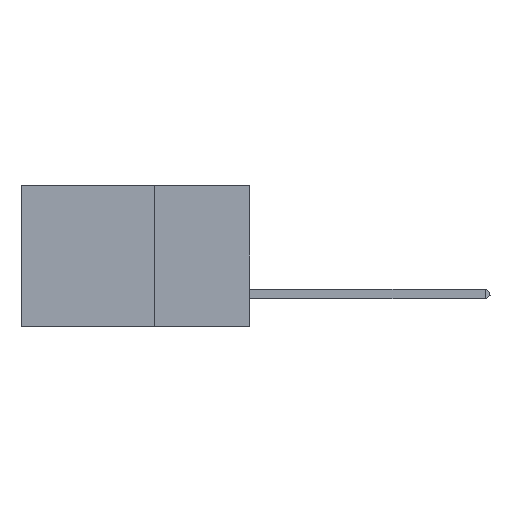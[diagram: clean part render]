
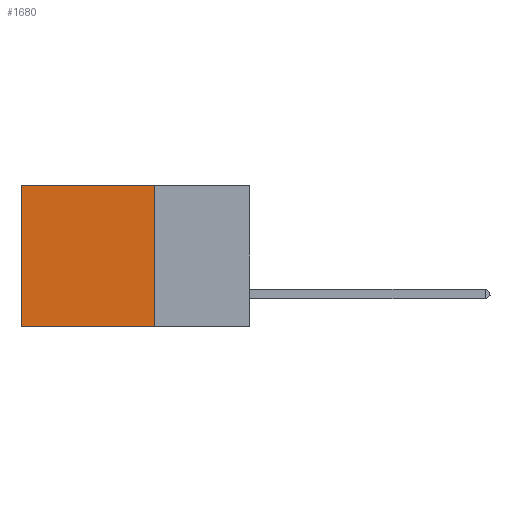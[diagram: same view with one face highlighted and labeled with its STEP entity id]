
A CAD part, left-side view. The second image highlights one B-rep face of the part: STEP entity #1680.
In plain terms, the highlighted planar face has unit normal (-1, 0, 0).
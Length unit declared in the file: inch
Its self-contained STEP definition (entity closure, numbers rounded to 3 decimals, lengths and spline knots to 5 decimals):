
#874 = ORIENTED_EDGE ( 'NONE', *, *, #21182, .F. ) ;
#1271 = CARTESIAN_POINT ( 'NONE',  ( 0.2875, 0.25, 0. ) ) ;
#1680 = ADVANCED_FACE ( 'NONE', ( #31434 ), #6539, .F. ) ;
#3953 = CARTESIAN_POINT ( 'NONE',  ( 0.2875, 0.25, 0. ) ) ;
#4051 = VERTEX_POINT ( 'NONE', #11781 ) ;
#4622 = EDGE_CURVE ( 'NONE', #23610, #4051, #10595, .T. ) ;
#5196 = CARTESIAN_POINT ( 'NONE',  ( 0.2875, 0.25, -0.37 ) ) ;
#5787 = VERTEX_POINT ( 'NONE', #28684 ) ;
#5851 = EDGE_CURVE ( 'NONE', #18109, #5787, #27146, .T. ) ;
#6539 = PLANE ( 'NONE',  #11853 ) ;
#6993 = LINE ( 'NONE', #5196, #16858 ) ;
#8782 = DIRECTION ( 'NONE',  ( 0., 0., -1. ) ) ;
#9508 = DIRECTION ( 'NONE',  ( 1., 0., 0. ) ) ;
#9754 = DIRECTION ( 'NONE',  ( 0., 0., -1. ) ) ;
#10595 = LINE ( 'NONE', #11895, #27715 ) ;
#11781 = CARTESIAN_POINT ( 'NONE',  ( 0.2875, 0.6, -0.37 ) ) ;
#11853 = AXIS2_PLACEMENT_3D ( 'NONE', #1271, #9508, #9754 ) ;
#11895 = CARTESIAN_POINT ( 'NONE',  ( 0.2875, 0.6, 0. ) ) ;
#13085 = DIRECTION ( 'NONE',  ( 0., 1., 0. ) ) ;
#13826 = CARTESIAN_POINT ( 'NONE',  ( 0.2875, 0.25, 0. ) ) ;
#16858 = VECTOR ( 'NONE', #25424, 39.37008 ) ;
#17115 = ORIENTED_EDGE ( 'NONE', *, *, #5851, .F. ) ;
#18109 = VERTEX_POINT ( 'NONE', #27267 ) ;
#21182 = EDGE_CURVE ( 'NONE', #5787, #4051, #6993, .T. ) ;
#23333 = CARTESIAN_POINT ( 'NONE',  ( 0.2875, 0.6, 0. ) ) ;
#23610 = VERTEX_POINT ( 'NONE', #23333 ) ;
#23626 = DIRECTION ( 'NONE',  ( 0., 0., -1. ) ) ;
#23820 = EDGE_CURVE ( 'NONE', #18109, #23610, #27064, .T. ) ;
#25424 = DIRECTION ( 'NONE',  ( 0., 1., 0. ) ) ;
#27064 = LINE ( 'NONE', #3953, #34704 ) ;
#27146 = LINE ( 'NONE', #13826, #34357 ) ;
#27267 = CARTESIAN_POINT ( 'NONE',  ( 0.2875, 0.25, 0. ) ) ;
#27715 = VECTOR ( 'NONE', #23626, 39.37008 ) ;
#28684 = CARTESIAN_POINT ( 'NONE',  ( 0.2875, 0.25, -0.37 ) ) ;
#30931 = EDGE_LOOP ( 'NONE', ( #33659, #874, #17115, #35596 ) ) ;
#31434 = FACE_OUTER_BOUND ( 'NONE', #30931, .T. ) ;
#33659 = ORIENTED_EDGE ( 'NONE', *, *, #4622, .T. ) ;
#34357 = VECTOR ( 'NONE', #8782, 39.37008 ) ;
#34704 = VECTOR ( 'NONE', #13085, 39.37008 ) ;
#35596 = ORIENTED_EDGE ( 'NONE', *, *, #23820, .T. ) ;
